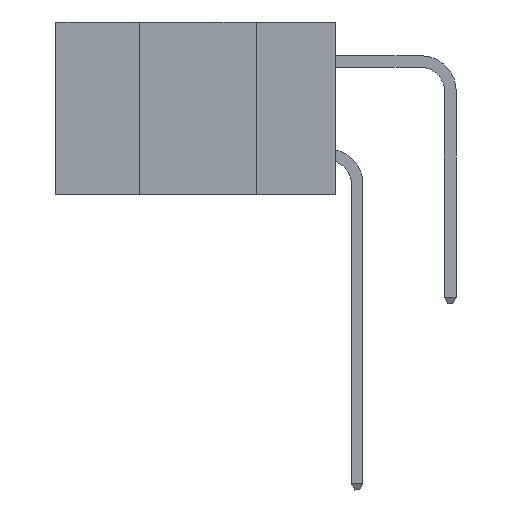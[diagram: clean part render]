
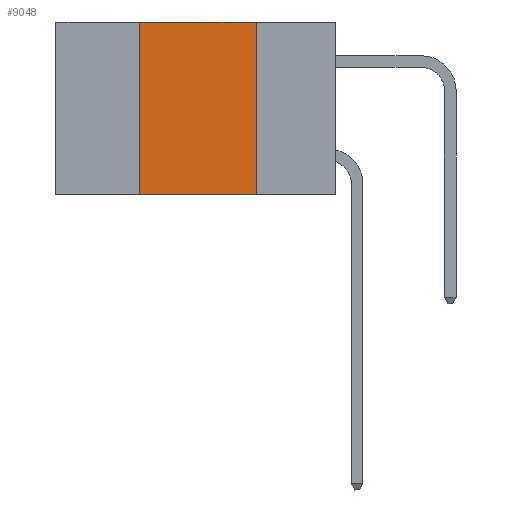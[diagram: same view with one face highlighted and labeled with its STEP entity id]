
A CAD part, left-side view. The second image highlights one B-rep face of the part: STEP entity #9048.
In plain terms, the highlighted planar face has unit normal (-1, 0, 0).
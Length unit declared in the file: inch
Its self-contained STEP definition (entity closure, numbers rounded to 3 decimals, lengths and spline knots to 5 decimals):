
#127 = LINE ( 'NONE', #7281, #10072 ) ;
#1035 = LINE ( 'NONE', #10467, #18278 ) ;
#1156 = CARTESIAN_POINT ( 'NONE',  ( 0., 0.17, 0. ) ) ;
#1733 = LINE ( 'NONE', #18162, #4351 ) ;
#1974 = FACE_OUTER_BOUND ( 'NONE', #6288, .T. ) ;
#2701 = CARTESIAN_POINT ( 'NONE',  ( 0., 0.6, 0. ) ) ;
#2705 = VERTEX_POINT ( 'NONE', #6859 ) ;
#4167 = PLANE ( 'NONE',  #7733 ) ;
#4351 = VECTOR ( 'NONE', #16713, 39.37008 ) ;
#4392 = DIRECTION ( 'NONE',  ( 0., 0., -1. ) ) ;
#5850 = DIRECTION ( 'NONE',  ( 0., -1., 0. ) ) ;
#6190 = EDGE_CURVE ( 'NONE', #13975, #2705, #1733, .T. ) ;
#6288 = EDGE_LOOP ( 'NONE', ( #21202, #6325, #14582, #20898 ) ) ;
#6296 = EDGE_CURVE ( 'NONE', #13975, #12049, #127, .T. ) ;
#6325 = ORIENTED_EDGE ( 'NONE', *, *, #7921, .F. ) ;
#6859 = CARTESIAN_POINT ( 'NONE',  ( 0., 0.42, 0. ) ) ;
#7281 = CARTESIAN_POINT ( 'NONE',  ( 0., 0.6, -0.37 ) ) ;
#7633 = LINE ( 'NONE', #20329, #20460 ) ;
#7733 = AXIS2_PLACEMENT_3D ( 'NONE', #2701, #12531, #4392 ) ;
#7921 = EDGE_CURVE ( 'NONE', #2705, #19332, #7633, .T. ) ;
#9048 = ADVANCED_FACE ( 'NONE', ( #1974 ), #4167, .F. ) ;
#10072 = VECTOR ( 'NONE', #5850, 39.37008 ) ;
#10311 = DIRECTION ( 'NONE',  ( 0., -1., 0. ) ) ;
#10467 = CARTESIAN_POINT ( 'NONE',  ( 0., 0.17, 0. ) ) ;
#12049 = VERTEX_POINT ( 'NONE', #18956 ) ;
#12130 = DIRECTION ( 'NONE',  ( 0., 0., -1. ) ) ;
#12531 = DIRECTION ( 'NONE',  ( 1., 0., 0. ) ) ;
#12605 = CARTESIAN_POINT ( 'NONE',  ( 0., 0.42, -0.37 ) ) ;
#13118 = EDGE_CURVE ( 'NONE', #19332, #12049, #1035, .T. ) ;
#13975 = VERTEX_POINT ( 'NONE', #12605 ) ;
#14582 = ORIENTED_EDGE ( 'NONE', *, *, #6190, .F. ) ;
#16713 = DIRECTION ( 'NONE',  ( 0., 0., 1. ) ) ;
#18162 = CARTESIAN_POINT ( 'NONE',  ( 0., 0.42, 0. ) ) ;
#18278 = VECTOR ( 'NONE', #12130, 39.37008 ) ;
#18956 = CARTESIAN_POINT ( 'NONE',  ( 0., 0.17, -0.37 ) ) ;
#19332 = VERTEX_POINT ( 'NONE', #1156 ) ;
#20329 = CARTESIAN_POINT ( 'NONE',  ( 0., 0.6, 0. ) ) ;
#20460 = VECTOR ( 'NONE', #10311, 39.37008 ) ;
#20898 = ORIENTED_EDGE ( 'NONE', *, *, #6296, .T. ) ;
#21202 = ORIENTED_EDGE ( 'NONE', *, *, #13118, .F. ) ;
